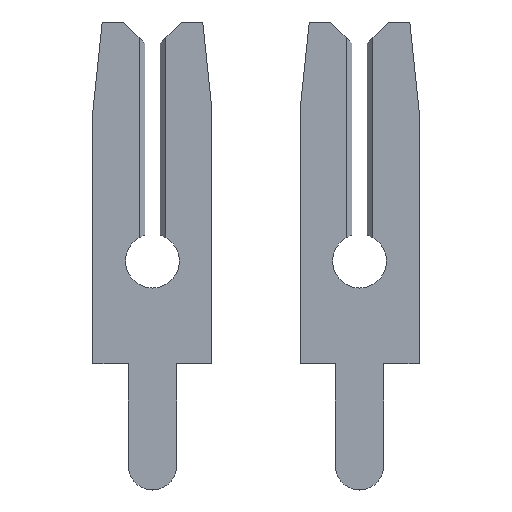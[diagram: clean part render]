
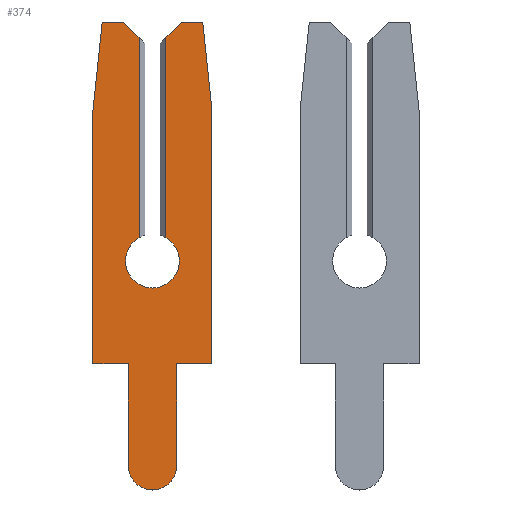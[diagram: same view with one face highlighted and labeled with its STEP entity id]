
A CAD part, top view. The second image highlights one B-rep face of the part: STEP entity #374.
In plain terms, the highlighted face is planar.
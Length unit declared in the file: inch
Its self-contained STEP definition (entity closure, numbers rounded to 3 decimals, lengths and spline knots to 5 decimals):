
#1 = EDGE_CURVE ( 'NONE', #894, #799, #550, .T. ) ;
#5 = CARTESIAN_POINT ( 'NONE',  ( -0.013, -0.099, 0.0575 ) ) ;
#24 = VERTEX_POINT ( 'NONE', #285 ) ;
#26 = LINE ( 'NONE', #282, #204 ) ;
#27 = EDGE_CURVE ( 'NONE', #441, #194, #26, .T. ) ;
#39 = CARTESIAN_POINT ( 'NONE',  ( -0.013, 0., 0. ) ) ;
#41 = LINE ( 'NONE', #166, #910 ) ;
#45 = ORIENTED_EDGE ( 'NONE', *, *, #354, .F. ) ;
#48 = ORIENTED_EDGE ( 'NONE', *, *, #138, .F. ) ;
#55 = EDGE_CURVE ( 'NONE', #841, #376, #915, .T. ) ;
#58 = DIRECTION ( 'NONE',  ( 0., 1., 0. ) ) ;
#61 = CARTESIAN_POINT ( 'NONE',  ( -0.013, -0.1975, -0.0235 ) ) ;
#72 = VERTEX_POINT ( 'NONE', #549 ) ;
#77 = ORIENTED_EDGE ( 'NONE', *, *, #27, .F. ) ;
#86 = LINE ( 'NONE', #762, #559 ) ;
#88 = EDGE_CURVE ( 'NONE', #588, #24, #356, .T. ) ;
#90 = CARTESIAN_POINT ( 'NONE',  ( -0.013, 0.2105, 0.0075 ) ) ;
#92 = VECTOR ( 'NONE', #189, 39.37008 ) ;
#100 = EDGE_CURVE ( 'NONE', #457, #72, #659, .T. ) ;
#101 = VERTEX_POINT ( 'NONE', #472 ) ;
#105 = CIRCLE ( 'NONE', #623, 0.0235 ) ;
#107 = EDGE_CURVE ( 'NONE', #72, #755, #410, .T. ) ;
#122 = CARTESIAN_POINT ( 'NONE',  ( -0.013, 0.231, 0.028 ) ) ;
#125 = VECTOR ( 'NONE', #367, 39.37008 ) ;
#128 = EDGE_CURVE ( 'NONE', #662, #140, #853, .T. ) ;
#132 = LINE ( 'NONE', #788, #476 ) ;
#133 = CARTESIAN_POINT ( 'NONE',  ( -0.013, -0.099, -0.0575 ) ) ;
#135 = DIRECTION ( 'NONE',  ( 0., -1., 0. ) ) ;
#138 = EDGE_CURVE ( 'NONE', #826, #997, #86, .T. ) ;
#140 = VERTEX_POINT ( 'NONE', #462 ) ;
#154 = DIRECTION ( 'NONE',  ( 0., 0., -1. ) ) ;
#166 = CARTESIAN_POINT ( 'NONE',  ( -0.013, 0.146, 0.0575 ) ) ;
#171 = DIRECTION ( 'NONE',  ( 1., 0., 0. ) ) ;
#176 = LINE ( 'NONE', #122, #343 ) ;
#183 = EDGE_CURVE ( 'NONE', #755, #841, #132, .T. ) ;
#189 = DIRECTION ( 'NONE',  ( 0., 0., -1. ) ) ;
#190 = CARTESIAN_POINT ( 'NONE',  ( -0.013, 0.216, 0.013 ) ) ;
#194 = VERTEX_POINT ( 'NONE', #325 ) ;
#195 = DIRECTION ( 'NONE',  ( 0., -0.707, 0.707 ) ) ;
#200 = EDGE_CURVE ( 'NONE', #194, #894, #105, .T. ) ;
#204 = VECTOR ( 'NONE', #135, 39.37008 ) ;
#205 = DIRECTION ( 'NONE',  ( 0., 0., 1. ) ) ;
#224 = DIRECTION ( 'NONE',  ( 0., 0., -1. ) ) ;
#228 = DIRECTION ( 'NONE',  ( 0., -0.995, 0.105 ) ) ;
#237 = DIRECTION ( 'NONE',  ( -1., 0., 0. ) ) ;
#242 = CARTESIAN_POINT ( 'NONE',  ( -0.013, -0.1975, 0. ) ) ;
#243 = LINE ( 'NONE', #270, #92 ) ;
#258 = LINE ( 'NONE', #90, #364 ) ;
#270 = CARTESIAN_POINT ( 'NONE',  ( -0.013, -0.099, -0.0575 ) ) ;
#279 = EDGE_CURVE ( 'NONE', #997, #457, #388, .T. ) ;
#282 = CARTESIAN_POINT ( 'NONE',  ( -0.013, -0.099, 0.0235 ) ) ;
#285 = CARTESIAN_POINT ( 'NONE',  ( -0.013, 0.146, 0.0575 ) ) ;
#291 = LINE ( 'NONE', #300, #125 ) ;
#296 = EDGE_LOOP ( 'NONE', ( #937, #464, #871, #358, #322, #987, #674, #768, #48, #45, #975, #556, #77, #818, #652, #889, #673, #780 ) ) ;
#297 = DIRECTION ( 'NONE',  ( 0., 1., 0. ) ) ;
#300 = CARTESIAN_POINT ( 'NONE',  ( -0.013, 0.231, 0.013 ) ) ;
#302 = CARTESIAN_POINT ( 'NONE',  ( -0.013, 0., 0. ) ) ;
#307 = CARTESIAN_POINT ( 'NONE',  ( -0.013, 0.2105, -0.0075 ) ) ;
#313 = CARTESIAN_POINT ( 'NONE',  ( -0.013, 0.231, -0.028 ) ) ;
#316 = DIRECTION ( 'NONE',  ( 0., 0.707, 0.707 ) ) ;
#320 = CARTESIAN_POINT ( 'NONE',  ( -0.013, 0., 0. ) ) ;
#321 = AXIS2_PLACEMENT_3D ( 'NONE', #39, #958, #804 ) ;
#322 = ORIENTED_EDGE ( 'NONE', *, *, #183, .F. ) ;
#325 = CARTESIAN_POINT ( 'NONE',  ( -0.013, -0.1975, 0.0235 ) ) ;
#342 = LINE ( 'NONE', #980, #969 ) ;
#343 = VECTOR ( 'NONE', #205, 39.37008 ) ;
#344 = CARTESIAN_POINT ( 'NONE',  ( -0.013, 0.231, -0.04857 ) ) ;
#354 = EDGE_CURVE ( 'NONE', #799, #826, #243, .T. ) ;
#356 = LINE ( 'NONE', #777, #459 ) ;
#358 = ORIENTED_EDGE ( 'NONE', *, *, #55, .F. ) ;
#359 = CARTESIAN_POINT ( 'NONE',  ( -0.013, -0.099, -0.0235 ) ) ;
#364 = VECTOR ( 'NONE', #316, 39.37008 ) ;
#367 = DIRECTION ( 'NONE',  ( 0., -1., 0. ) ) ;
#374 = ADVANCED_FACE ( 'NONE', ( #971 ), #947, .F. ) ;
#375 = CARTESIAN_POINT ( 'NONE',  ( -0.013, -0.099, -0.0235 ) ) ;
#376 = VERTEX_POINT ( 'NONE', #637 ) ;
#388 = LINE ( 'NONE', #861, #791 ) ;
#396 = DIRECTION ( 'NONE',  ( 0., 0., 1. ) ) ;
#410 = LINE ( 'NONE', #307, #901 ) ;
#419 = AXIS2_PLACEMENT_3D ( 'NONE', #320, #995, #154 ) ;
#431 = CIRCLE ( 'NONE', #419, 0.026 ) ;
#441 = VERTEX_POINT ( 'NONE', #661 ) ;
#449 = VERTEX_POINT ( 'NONE', #190 ) ;
#457 = VERTEX_POINT ( 'NONE', #344 ) ;
#459 = VECTOR ( 'NONE', #228, 39.37008 ) ;
#462 = CARTESIAN_POINT ( 'NONE',  ( -0.013, 0.02252, 0.013 ) ) ;
#463 = AXIS2_PLACEMENT_3D ( 'NONE', #632, #237, #701 ) ;
#464 = ORIENTED_EDGE ( 'NONE', *, *, #128, .F. ) ;
#472 = CARTESIAN_POINT ( 'NONE',  ( -0.013, 0.231, 0.028 ) ) ;
#476 = VECTOR ( 'NONE', #648, 39.37008 ) ;
#514 = CARTESIAN_POINT ( 'NONE',  ( -0.013, 0.231, 0.04857 ) ) ;
#548 = DIRECTION ( 'NONE',  ( 0., -1., 0. ) ) ;
#549 = CARTESIAN_POINT ( 'NONE',  ( -0.013, 0.231, -0.028 ) ) ;
#550 = LINE ( 'NONE', #359, #600 ) ;
#556 = ORIENTED_EDGE ( 'NONE', *, *, #200, .F. ) ;
#559 = VECTOR ( 'NONE', #297, 39.37008 ) ;
#564 = DIRECTION ( 'NONE',  ( 0., 0.995, 0.105 ) ) ;
#583 = EDGE_CURVE ( 'NONE', #101, #588, #176, .T. ) ;
#588 = VERTEX_POINT ( 'NONE', #514 ) ;
#600 = VECTOR ( 'NONE', #58, 39.37008 ) ;
#623 = AXIS2_PLACEMENT_3D ( 'NONE', #242, #171, #864 ) ;
#632 = CARTESIAN_POINT ( 'NONE',  ( -0.013, 0., 0. ) ) ;
#637 = CARTESIAN_POINT ( 'NONE',  ( -0.013, 0., -0.026 ) ) ;
#648 = DIRECTION ( 'NONE',  ( 0., -1., 0. ) ) ;
#652 = ORIENTED_EDGE ( 'NONE', *, *, #929, .F. ) ;
#657 = AXIS2_PLACEMENT_3D ( 'NONE', #302, #690, #224 ) ;
#659 = LINE ( 'NONE', #313, #934 ) ;
#661 = CARTESIAN_POINT ( 'NONE',  ( -0.013, -0.099, 0.0235 ) ) ;
#662 = VERTEX_POINT ( 'NONE', #899 ) ;
#673 = ORIENTED_EDGE ( 'NONE', *, *, #583, .F. ) ;
#674 = ORIENTED_EDGE ( 'NONE', *, *, #100, .F. ) ;
#678 = CARTESIAN_POINT ( 'NONE',  ( -0.013, 0.216, -0.013 ) ) ;
#686 = CARTESIAN_POINT ( 'NONE',  ( -0.013, 0.02252, -0.013 ) ) ;
#690 = DIRECTION ( 'NONE',  ( -1., 0., 0. ) ) ;
#699 = CARTESIAN_POINT ( 'NONE',  ( -0.013, 0.146, -0.0575 ) ) ;
#701 = DIRECTION ( 'NONE',  ( 0., 0., -1. ) ) ;
#754 = DIRECTION ( 'NONE',  ( 0., 0., -1. ) ) ;
#755 = VERTEX_POINT ( 'NONE', #678 ) ;
#762 = CARTESIAN_POINT ( 'NONE',  ( -0.013, 0.146, -0.0575 ) ) ;
#768 = ORIENTED_EDGE ( 'NONE', *, *, #279, .F. ) ;
#777 = CARTESIAN_POINT ( 'NONE',  ( -0.013, 0.231, 0.04857 ) ) ;
#780 = ORIENTED_EDGE ( 'NONE', *, *, #991, .F. ) ;
#788 = CARTESIAN_POINT ( 'NONE',  ( -0.013, 0., -0.013 ) ) ;
#791 = VECTOR ( 'NONE', #564, 39.37008 ) ;
#799 = VERTEX_POINT ( 'NONE', #375 ) ;
#804 = DIRECTION ( 'NONE',  ( 0., 0., -1. ) ) ;
#818 = ORIENTED_EDGE ( 'NONE', *, *, #881, .F. ) ;
#826 = VERTEX_POINT ( 'NONE', #133 ) ;
#834 = EDGE_CURVE ( 'NONE', #449, #140, #291, .T. ) ;
#841 = VERTEX_POINT ( 'NONE', #686 ) ;
#853 = CIRCLE ( 'NONE', #657, 0.026 ) ;
#861 = CARTESIAN_POINT ( 'NONE',  ( -0.013, 0.231, -0.04857 ) ) ;
#864 = DIRECTION ( 'NONE',  ( 0., 0., 1. ) ) ;
#871 = ORIENTED_EDGE ( 'NONE', *, *, #994, .F. ) ;
#881 = EDGE_CURVE ( 'NONE', #983, #441, #342, .T. ) ;
#889 = ORIENTED_EDGE ( 'NONE', *, *, #88, .F. ) ;
#894 = VERTEX_POINT ( 'NONE', #61 ) ;
#899 = CARTESIAN_POINT ( 'NONE',  ( -0.013, 0., 0.026 ) ) ;
#901 = VECTOR ( 'NONE', #195, 39.37008 ) ;
#910 = VECTOR ( 'NONE', #548, 39.37008 ) ;
#915 = CIRCLE ( 'NONE', #463, 0.026 ) ;
#929 = EDGE_CURVE ( 'NONE', #24, #983, #41, .T. ) ;
#934 = VECTOR ( 'NONE', #396, 39.37008 ) ;
#937 = ORIENTED_EDGE ( 'NONE', *, *, #834, .T. ) ;
#947 = PLANE ( 'NONE',  #321 ) ;
#958 = DIRECTION ( 'NONE',  ( 1., 0., 0. ) ) ;
#969 = VECTOR ( 'NONE', #754, 39.37008 ) ;
#971 = FACE_OUTER_BOUND ( 'NONE', #296, .T. ) ;
#975 = ORIENTED_EDGE ( 'NONE', *, *, #1, .F. ) ;
#980 = CARTESIAN_POINT ( 'NONE',  ( -0.013, -0.099, 0.0575 ) ) ;
#983 = VERTEX_POINT ( 'NONE', #5 ) ;
#987 = ORIENTED_EDGE ( 'NONE', *, *, #107, .F. ) ;
#991 = EDGE_CURVE ( 'NONE', #449, #101, #258, .T. ) ;
#994 = EDGE_CURVE ( 'NONE', #376, #662, #431, .T. ) ;
#995 = DIRECTION ( 'NONE',  ( -1., 0., 0. ) ) ;
#997 = VERTEX_POINT ( 'NONE', #699 ) ;
